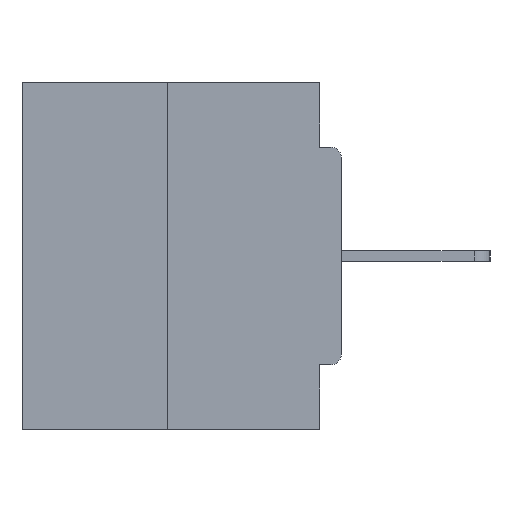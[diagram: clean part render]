
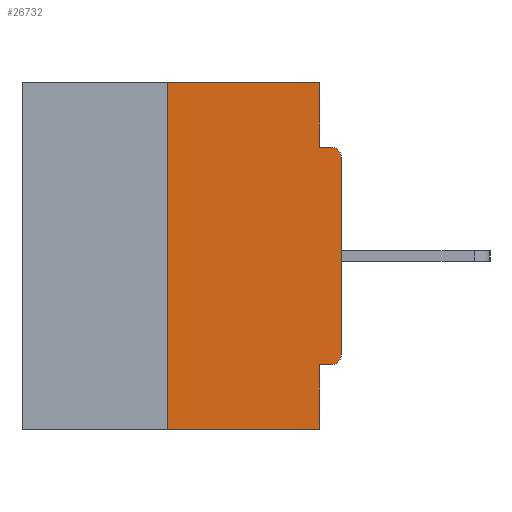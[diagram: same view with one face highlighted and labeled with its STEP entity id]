
A CAD part, left-side view. The second image highlights one B-rep face of the part: STEP entity #26732.
In plain terms, the highlighted planar face has unit normal (-1, 0, 0).
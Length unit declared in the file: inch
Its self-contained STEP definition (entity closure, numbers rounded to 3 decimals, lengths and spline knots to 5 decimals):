
#414 = ORIENTED_EDGE ( 'NONE', *, *, #3076, .F. ) ;
#504 = EDGE_CURVE ( 'NONE', #22956, #4716, #25062, .T. ) ;
#761 = LINE ( 'NONE', #17839, #30666 ) ;
#1895 = LINE ( 'NONE', #14921, #8799 ) ;
#2130 = ORIENTED_EDGE ( 'NONE', *, *, #6647, .T. ) ;
#3076 = EDGE_CURVE ( 'NONE', #15495, #7038, #3523, .T. ) ;
#3523 = LINE ( 'NONE', #7000, #32468 ) ;
#3923 = DIRECTION ( 'NONE',  ( 0., 0., -1. ) ) ;
#4529 = VERTEX_POINT ( 'NONE', #4656 ) ;
#4603 = LINE ( 'NONE', #19651, #10332 ) ;
#4656 = CARTESIAN_POINT ( 'NONE',  ( 0., 0., -0.1085 ) ) ;
#4716 = VERTEX_POINT ( 'NONE', #9187 ) ;
#4933 = DIRECTION ( 'NONE',  ( 0., -1., 0. ) ) ;
#5266 = CIRCLE ( 'NONE', #13786, 0.015 ) ;
#5822 = AXIS2_PLACEMENT_3D ( 'NONE', #29064, #24348, #3923 ) ;
#6206 = ORIENTED_EDGE ( 'NONE', *, *, #28205, .F. ) ;
#6647 = EDGE_CURVE ( 'NONE', #4716, #4529, #23097, .T. ) ;
#6764 = VECTOR ( 'NONE', #9762, 39.37008 ) ;
#7000 = CARTESIAN_POINT ( 'NONE',  ( 0., 0.031, 0. ) ) ;
#7038 = VERTEX_POINT ( 'NONE', #30293 ) ;
#7272 = CARTESIAN_POINT ( 'NONE',  ( 0., 0.031, -0.4065 ) ) ;
#7316 = EDGE_CURVE ( 'NONE', #17204, #18760, #19780, .T. ) ;
#7463 = DIRECTION ( 'NONE',  ( 0., -1., 0. ) ) ;
#7815 = DIRECTION ( 'NONE',  ( 0., 0., -1. ) ) ;
#7988 = DIRECTION ( 'NONE',  ( 0., 1., 0. ) ) ;
#8459 = ORIENTED_EDGE ( 'NONE', *, *, #504, .T. ) ;
#8799 = VECTOR ( 'NONE', #12091, 39.37008 ) ;
#8803 = FACE_OUTER_BOUND ( 'NONE', #22395, .T. ) ;
#8902 = EDGE_CURVE ( 'NONE', #4529, #22142, #5266, .T. ) ;
#9187 = CARTESIAN_POINT ( 'NONE',  ( 0., 0., -0.3915 ) ) ;
#9505 = VECTOR ( 'NONE', #15703, 39.37008 ) ;
#9762 = DIRECTION ( 'NONE',  ( 0., -1., 0. ) ) ;
#9785 = ORIENTED_EDGE ( 'NONE', *, *, #16208, .F. ) ;
#10332 = VECTOR ( 'NONE', #4933, 39.37008 ) ;
#10365 = CARTESIAN_POINT ( 'NONE',  ( 0., 0., 0. ) ) ;
#10483 = LINE ( 'NONE', #20701, #18906 ) ;
#11061 = CARTESIAN_POINT ( 'NONE',  ( 0., 0.015, -0.4065 ) ) ;
#12091 = DIRECTION ( 'NONE',  ( 0., 0., 1. ) ) ;
#12534 = CARTESIAN_POINT ( 'NONE',  ( 0., 0.015, -0.0935 ) ) ;
#12587 = CARTESIAN_POINT ( 'NONE',  ( 0., 0.46, -0.5 ) ) ;
#12633 = VERTEX_POINT ( 'NONE', #7272 ) ;
#13786 = AXIS2_PLACEMENT_3D ( 'NONE', #18463, #29036, #28710 ) ;
#13878 = DIRECTION ( 'NONE',  ( 0., 0., -1. ) ) ;
#14918 = EDGE_CURVE ( 'NONE', #12633, #18760, #761, .T. ) ;
#14921 = CARTESIAN_POINT ( 'NONE',  ( 0., 0.25, 0. ) ) ;
#15201 = EDGE_CURVE ( 'NONE', #32662, #15495, #4603, .T. ) ;
#15495 = VERTEX_POINT ( 'NONE', #26835 ) ;
#15703 = DIRECTION ( 'NONE',  ( 0., 0., 1. ) ) ;
#16208 = EDGE_CURVE ( 'NONE', #22956, #12633, #10483, .T. ) ;
#16870 = ORIENTED_EDGE ( 'NONE', *, *, #14918, .F. ) ;
#16894 = EDGE_CURVE ( 'NONE', #17204, #32662, #1895, .T. ) ;
#17204 = VERTEX_POINT ( 'NONE', #26315 ) ;
#17385 = AXIS2_PLACEMENT_3D ( 'NONE', #18673, #24357, #26884 ) ;
#17839 = CARTESIAN_POINT ( 'NONE',  ( 0., 0.031, -0.5 ) ) ;
#18463 = CARTESIAN_POINT ( 'NONE',  ( 0., 0.015, -0.1085 ) ) ;
#18673 = CARTESIAN_POINT ( 'NONE',  ( 0., 0.46, 0. ) ) ;
#18760 = VERTEX_POINT ( 'NONE', #29725 ) ;
#18906 = VECTOR ( 'NONE', #7988, 39.37008 ) ;
#19651 = CARTESIAN_POINT ( 'NONE',  ( 0., 0.46, 0. ) ) ;
#19780 = LINE ( 'NONE', #12587, #6764 ) ;
#20701 = CARTESIAN_POINT ( 'NONE',  ( 0., 0., -0.4065 ) ) ;
#22142 = VERTEX_POINT ( 'NONE', #12534 ) ;
#22395 = EDGE_LOOP ( 'NONE', ( #26199, #28862, #25659, #16870, #9785, #8459, #2130, #30573, #6206, #414 ) ) ;
#22956 = VERTEX_POINT ( 'NONE', #11061 ) ;
#23097 = LINE ( 'NONE', #10365, #9505 ) ;
#24348 = DIRECTION ( 'NONE',  ( -1., 0., 0. ) ) ;
#24357 = DIRECTION ( 'NONE',  ( 1., 0., 0. ) ) ;
#24696 = CARTESIAN_POINT ( 'NONE',  ( 0., 0.25, 0. ) ) ;
#25062 = CIRCLE ( 'NONE', #5822, 0.015 ) ;
#25206 = CARTESIAN_POINT ( 'NONE',  ( 0., 0., -0.0935 ) ) ;
#25659 = ORIENTED_EDGE ( 'NONE', *, *, #7316, .T. ) ;
#26199 = ORIENTED_EDGE ( 'NONE', *, *, #15201, .F. ) ;
#26315 = CARTESIAN_POINT ( 'NONE',  ( 0., 0.25, -0.5 ) ) ;
#26732 = ADVANCED_FACE ( 'NONE', ( #8803 ), #31600, .F. ) ;
#26835 = CARTESIAN_POINT ( 'NONE',  ( 0., 0.031, 0. ) ) ;
#26884 = DIRECTION ( 'NONE',  ( 0., 0., -1. ) ) ;
#27553 = LINE ( 'NONE', #25206, #28717 ) ;
#28205 = EDGE_CURVE ( 'NONE', #7038, #22142, #27553, .T. ) ;
#28710 = DIRECTION ( 'NONE',  ( 0., 0., -1. ) ) ;
#28717 = VECTOR ( 'NONE', #7463, 39.37008 ) ;
#28862 = ORIENTED_EDGE ( 'NONE', *, *, #16894, .F. ) ;
#29036 = DIRECTION ( 'NONE',  ( -1., 0., 0. ) ) ;
#29064 = CARTESIAN_POINT ( 'NONE',  ( 0., 0.015, -0.3915 ) ) ;
#29725 = CARTESIAN_POINT ( 'NONE',  ( 0., 0.031, -0.5 ) ) ;
#30293 = CARTESIAN_POINT ( 'NONE',  ( 0., 0.031, -0.0935 ) ) ;
#30573 = ORIENTED_EDGE ( 'NONE', *, *, #8902, .T. ) ;
#30666 = VECTOR ( 'NONE', #7815, 39.37008 ) ;
#31600 = PLANE ( 'NONE',  #17385 ) ;
#32468 = VECTOR ( 'NONE', #13878, 39.37008 ) ;
#32662 = VERTEX_POINT ( 'NONE', #24696 ) ;
